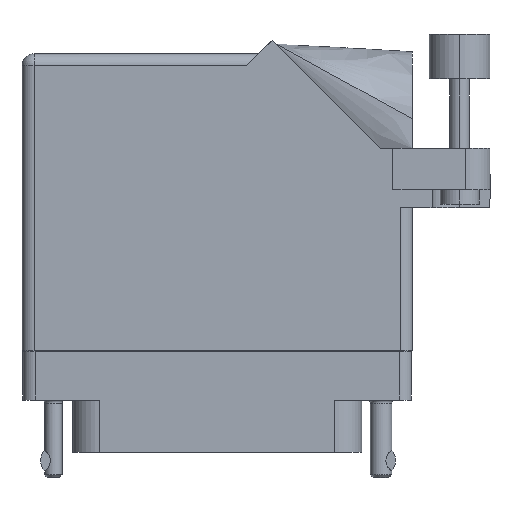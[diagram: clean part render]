
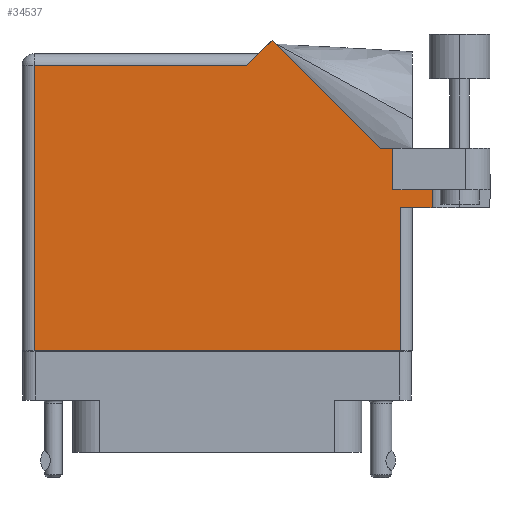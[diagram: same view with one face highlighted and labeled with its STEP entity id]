
A CAD part, front view. The second image highlights one B-rep face of the part: STEP entity #34537.
In plain terms, the highlighted face is planar.
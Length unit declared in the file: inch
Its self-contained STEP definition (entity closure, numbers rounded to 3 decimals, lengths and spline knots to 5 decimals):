
#974 = CARTESIAN_POINT ( 'NONE',  ( -1.005, 1.368, 0.455 ) ) ;
#1121 = EDGE_CURVE ( 'NONE', #33659, #34033, #12014, .T. ) ;
#1456 = DIRECTION ( 'NONE',  ( -1., 0., 0. ) ) ;
#1586 = EDGE_CURVE ( 'NONE', #12936, #46800, #47929, .T. ) ;
#2325 = LINE ( 'NONE', #5591, #41269 ) ;
#2369 = LINE ( 'NONE', #9403, #22298 ) ;
#2399 = ORIENTED_EDGE ( 'NONE', *, *, #21094, .T. ) ;
#2520 = DIRECTION ( 'NONE',  ( 1., 0., 0. ) ) ;
#3206 = VECTOR ( 'NONE', #35138, 39.37008 ) ;
#3508 = EDGE_CURVE ( 'NONE', #8633, #33659, #20726, .T. ) ;
#5591 = CARTESIAN_POINT ( 'NONE',  ( 0.83942, 0.944, 0.455 ) ) ;
#6197 = FACE_OUTER_BOUND ( 'NONE', #14860, .T. ) ;
#7080 = CARTESIAN_POINT ( 'NONE',  ( 0.905, 0.731, 0.455 ) ) ;
#7182 = CARTESIAN_POINT ( 'NONE',  ( 0.905, 0.731, 0.455 ) ) ;
#7915 = ORIENTED_EDGE ( 'NONE', *, *, #1121, .F. ) ;
#8080 = CARTESIAN_POINT ( 'NONE',  ( 0.83942, 0.944, 0.455 ) ) ;
#8463 = EDGE_CURVE ( 'NONE', #12027, #29836, #2325, .T. ) ;
#8633 = VERTEX_POINT ( 'NONE', #7080 ) ;
#9208 = VERTEX_POINT ( 'NONE', #14539 ) ;
#9403 = CARTESIAN_POINT ( 'NONE',  ( 0.212, 1.43, 0.455 ) ) ;
#10089 = DIRECTION ( 'NONE',  ( -0.707, 0.707, 0. ) ) ;
#10294 = LINE ( 'NONE', #17821, #41544 ) ;
#10834 = EDGE_CURVE ( 'NONE', #46800, #34033, #12135, .T. ) ;
#11639 = CARTESIAN_POINT ( 'NONE',  ( 1.005, 0.637, 0.455 ) ) ;
#12014 = LINE ( 'NONE', #27345, #3206 ) ;
#12027 = VERTEX_POINT ( 'NONE', #8080 ) ;
#12135 = LINE ( 'NONE', #11639, #25307 ) ;
#12922 = EDGE_CURVE ( 'NONE', #9208, #25985, #10294, .T. ) ;
#12936 = VERTEX_POINT ( 'NONE', #14548 ) ;
#13890 = DIRECTION ( 'NONE',  ( -1., 0., 0. ) ) ;
#14498 = VECTOR ( 'NONE', #13890, 39.37008 ) ;
#14539 = CARTESIAN_POINT ( 'NONE',  ( -0.943, 1.368, 0.455 ) ) ;
#14548 = CARTESIAN_POINT ( 'NONE',  ( 0.943, -0.1, 0.455 ) ) ;
#14804 = ORIENTED_EDGE ( 'NONE', *, *, #10834, .T. ) ;
#14805 = ORIENTED_EDGE ( 'NONE', *, *, #26212, .T. ) ;
#14860 = EDGE_LOOP ( 'NONE', ( #36097, #28141, #14804, #7915, #41444, #14805, #2399, #14868, #20425, #22103, #25335 ) ) ;
#14868 = ORIENTED_EDGE ( 'NONE', *, *, #8463, .T. ) ;
#17821 = CARTESIAN_POINT ( 'NONE',  ( -0.943, -0.1, 0.455 ) ) ;
#19278 = EDGE_CURVE ( 'NONE', #25985, #12936, #28884, .T. ) ;
#19854 = VERTEX_POINT ( 'NONE', #35199 ) ;
#20425 = ORIENTED_EDGE ( 'NONE', *, *, #45800, .T. ) ;
#20535 = CARTESIAN_POINT ( 'NONE',  ( 0.943, 0.637, 0.455 ) ) ;
#20700 = VECTOR ( 'NONE', #1456, 39.37008 ) ;
#20726 = LINE ( 'NONE', #25242, #47165 ) ;
#21094 = EDGE_CURVE ( 'NONE', #19854, #12027, #44776, .T. ) ;
#22103 = ORIENTED_EDGE ( 'NONE', *, *, #33081, .T. ) ;
#22117 = CARTESIAN_POINT ( 'NONE',  ( 1.1065, 0.731, 0.455 ) ) ;
#22298 = VECTOR ( 'NONE', #28994, 39.37008 ) ;
#23080 = CARTESIAN_POINT ( 'NONE',  ( 0.15, 1.368, 0.455 ) ) ;
#24759 = CARTESIAN_POINT ( 'NONE',  ( -0.943, -0.1, 0.455 ) ) ;
#24840 = CARTESIAN_POINT ( 'NONE',  ( 1.1065, 0.637, 0.455 ) ) ;
#25114 = CARTESIAN_POINT ( 'NONE',  ( -1.005, -0.1, 0.455 ) ) ;
#25242 = CARTESIAN_POINT ( 'NONE',  ( 0.905, 0.731, 0.455 ) ) ;
#25307 = VECTOR ( 'NONE', #46073, 39.37008 ) ;
#25335 = ORIENTED_EDGE ( 'NONE', *, *, #12922, .T. ) ;
#25513 = PLANE ( 'NONE',  #43949 ) ;
#25985 = VERTEX_POINT ( 'NONE', #24759 ) ;
#26212 = EDGE_CURVE ( 'NONE', #8633, #19854, #34807, .T. ) ;
#27345 = CARTESIAN_POINT ( 'NONE',  ( 1.1065, 1.06177, 0.455 ) ) ;
#27453 = VECTOR ( 'NONE', #2520, 39.37008 ) ;
#28141 = ORIENTED_EDGE ( 'NONE', *, *, #1586, .T. ) ;
#28884 = LINE ( 'NONE', #25114, #27453 ) ;
#28885 = VECTOR ( 'NONE', #38072, 39.37008 ) ;
#28994 = DIRECTION ( 'NONE',  ( -0.707, -0.707, 0. ) ) ;
#29272 = DIRECTION ( 'NONE',  ( 1., 0., 0. ) ) ;
#29836 = VERTEX_POINT ( 'NONE', #37194 ) ;
#31988 = DIRECTION ( 'NONE',  ( 0., -1., 0. ) ) ;
#33081 = EDGE_CURVE ( 'NONE', #44363, #9208, #47424, .T. ) ;
#33659 = VERTEX_POINT ( 'NONE', #22117 ) ;
#34033 = VERTEX_POINT ( 'NONE', #24840 ) ;
#34537 = ADVANCED_FACE ( 'NONE', ( #6197 ), #25513, .F. ) ;
#34807 = LINE ( 'NONE', #7182, #28885 ) ;
#35138 = DIRECTION ( 'NONE',  ( 0., -1., 0. ) ) ;
#35199 = CARTESIAN_POINT ( 'NONE',  ( 0.905, 0.944, 0.455 ) ) ;
#36097 = ORIENTED_EDGE ( 'NONE', *, *, #19278, .T. ) ;
#37194 = CARTESIAN_POINT ( 'NONE',  ( 0.28271, 1.50071, 0.455 ) ) ;
#37334 = DIRECTION ( 'NONE',  ( 0., 0., -1. ) ) ;
#38072 = DIRECTION ( 'NONE',  ( 0., 1., 0. ) ) ;
#39238 = CARTESIAN_POINT ( 'NONE',  ( 0.943, 0.637, 0.455 ) ) ;
#40844 = CARTESIAN_POINT ( 'NONE',  ( -1.005, 1.43, 0.455 ) ) ;
#41101 = DIRECTION ( 'NONE',  ( -1., 0., 0. ) ) ;
#41269 = VECTOR ( 'NONE', #10089, 39.37008 ) ;
#41444 = ORIENTED_EDGE ( 'NONE', *, *, #3508, .F. ) ;
#41544 = VECTOR ( 'NONE', #31988, 39.37008 ) ;
#43949 = AXIS2_PLACEMENT_3D ( 'NONE', #40844, #37334, #41101 ) ;
#44363 = VERTEX_POINT ( 'NONE', #23080 ) ;
#44776 = LINE ( 'NONE', #48326, #14498 ) ;
#45800 = EDGE_CURVE ( 'NONE', #29836, #44363, #2369, .T. ) ;
#46073 = DIRECTION ( 'NONE',  ( 1., 0., 0. ) ) ;
#46419 = VECTOR ( 'NONE', #48433, 39.37008 ) ;
#46800 = VERTEX_POINT ( 'NONE', #39238 ) ;
#47165 = VECTOR ( 'NONE', #29272, 39.37008 ) ;
#47424 = LINE ( 'NONE', #974, #20700 ) ;
#47929 = LINE ( 'NONE', #20535, #46419 ) ;
#48326 = CARTESIAN_POINT ( 'NONE',  ( 1.405, 0.944, 0.455 ) ) ;
#48433 = DIRECTION ( 'NONE',  ( 0., 1., 0. ) ) ;
